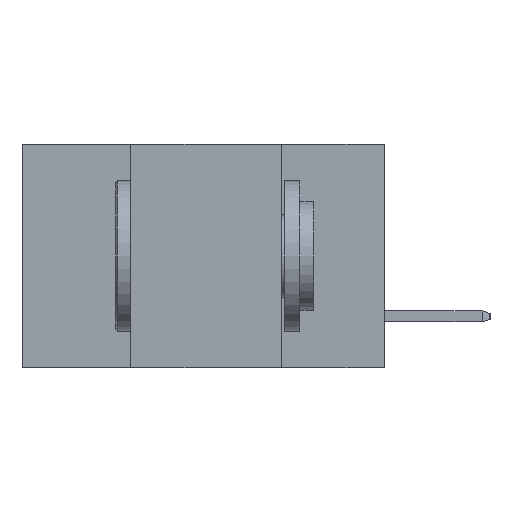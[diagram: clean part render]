
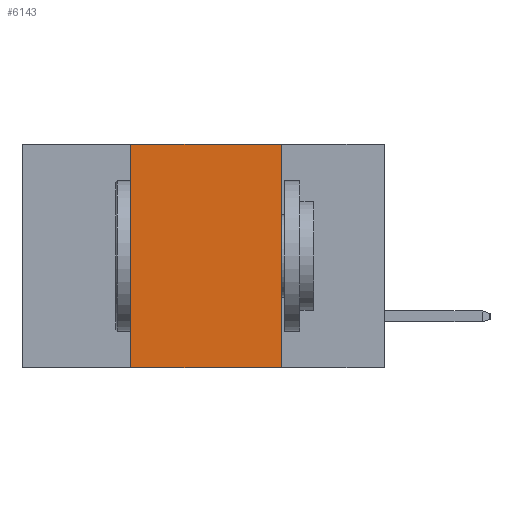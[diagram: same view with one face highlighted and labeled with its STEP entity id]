
A CAD part, left-side view. The second image highlights one B-rep face of the part: STEP entity #6143.
In plain terms, the highlighted planar face has unit normal (-1, 0, 0).
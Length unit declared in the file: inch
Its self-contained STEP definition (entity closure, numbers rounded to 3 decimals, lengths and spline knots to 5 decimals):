
#102 = EDGE_CURVE ( 'NONE', #10563, #9503, #11741, .T. ) ;
#1069 = VECTOR ( 'NONE', #22335, 39.37008 ) ;
#1953 = EDGE_LOOP ( 'NONE', ( #12112, #15886, #19759, #23503 ) ) ;
#4043 = VECTOR ( 'NONE', #25645, 39.37008 ) ;
#4606 = VECTOR ( 'NONE', #9272, 39.37008 ) ;
#6071 = LINE ( 'NONE', #14856, #21567 ) ;
#6143 = ADVANCED_FACE ( 'NONE', ( #13547 ), #8465, .F. ) ;
#8294 = DIRECTION ( 'NONE',  ( 0., 0., -1. ) ) ;
#8378 = DIRECTION ( 'NONE',  ( 1., 0., 0. ) ) ;
#8432 = CARTESIAN_POINT ( 'NONE',  ( 0., 0.6, 0. ) ) ;
#8465 = PLANE ( 'NONE',  #19947 ) ;
#9272 = DIRECTION ( 'NONE',  ( 0., 0., -1. ) ) ;
#9363 = LINE ( 'NONE', #13665, #4043 ) ;
#9503 = VERTEX_POINT ( 'NONE', #20521 ) ;
#10563 = VERTEX_POINT ( 'NONE', #18205 ) ;
#10830 = DIRECTION ( 'NONE',  ( 0., -1., 0. ) ) ;
#11741 = LINE ( 'NONE', #21999, #1069 ) ;
#11818 = VERTEX_POINT ( 'NONE', #20497 ) ;
#12112 = ORIENTED_EDGE ( 'NONE', *, *, #13561, .F. ) ;
#13547 = FACE_OUTER_BOUND ( 'NONE', #1953, .T. ) ;
#13561 = EDGE_CURVE ( 'NONE', #19802, #11818, #25912, .T. ) ;
#13665 = CARTESIAN_POINT ( 'NONE',  ( 0., 0.6, 0. ) ) ;
#14856 = CARTESIAN_POINT ( 'NONE',  ( 0., 0.6, -0.37 ) ) ;
#15236 = CARTESIAN_POINT ( 'NONE',  ( 0., 0.17, 0. ) ) ;
#15385 = EDGE_CURVE ( 'NONE', #10563, #11818, #6071, .T. ) ;
#15886 = ORIENTED_EDGE ( 'NONE', *, *, #19946, .F. ) ;
#18205 = CARTESIAN_POINT ( 'NONE',  ( 0., 0.42, -0.37 ) ) ;
#19359 = CARTESIAN_POINT ( 'NONE',  ( 0., 0.17, 0. ) ) ;
#19759 = ORIENTED_EDGE ( 'NONE', *, *, #102, .F. ) ;
#19802 = VERTEX_POINT ( 'NONE', #15236 ) ;
#19946 = EDGE_CURVE ( 'NONE', #9503, #19802, #9363, .T. ) ;
#19947 = AXIS2_PLACEMENT_3D ( 'NONE', #8432, #8378, #8294 ) ;
#20497 = CARTESIAN_POINT ( 'NONE',  ( 0., 0.17, -0.37 ) ) ;
#20521 = CARTESIAN_POINT ( 'NONE',  ( 0., 0.42, 0. ) ) ;
#21567 = VECTOR ( 'NONE', #10830, 39.37008 ) ;
#21999 = CARTESIAN_POINT ( 'NONE',  ( 0., 0.42, 0. ) ) ;
#22335 = DIRECTION ( 'NONE',  ( 0., 0., 1. ) ) ;
#23503 = ORIENTED_EDGE ( 'NONE', *, *, #15385, .T. ) ;
#25645 = DIRECTION ( 'NONE',  ( 0., -1., 0. ) ) ;
#25912 = LINE ( 'NONE', #19359, #4606 ) ;
